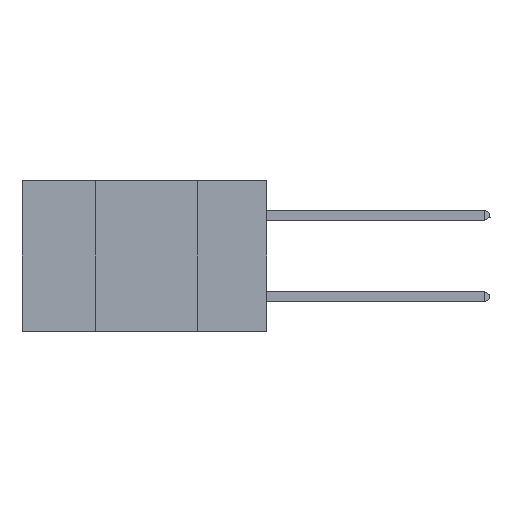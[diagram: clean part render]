
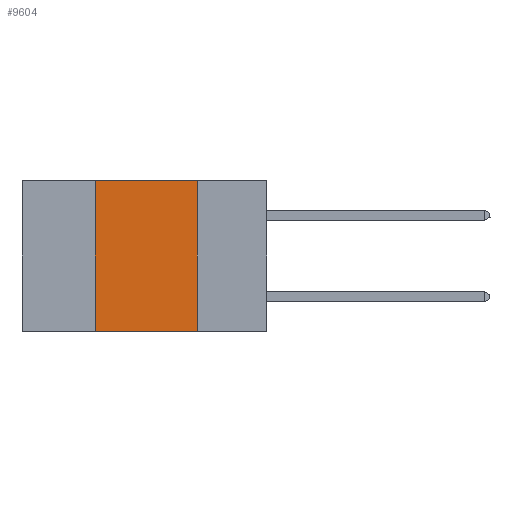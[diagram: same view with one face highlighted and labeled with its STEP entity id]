
A CAD part, left-side view. The second image highlights one B-rep face of the part: STEP entity #9604.
In plain terms, the highlighted planar face has unit normal (-1, 0, 0).
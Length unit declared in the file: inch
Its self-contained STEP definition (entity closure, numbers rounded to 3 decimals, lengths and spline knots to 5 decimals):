
#288 = CARTESIAN_POINT ( 'NONE',  ( 0., 0.6, -0.37 ) ) ;
#707 = VECTOR ( 'NONE', #19531, 39.37008 ) ;
#760 = CARTESIAN_POINT ( 'NONE',  ( 0., 0.17, -0.37 ) ) ;
#2148 = FACE_OUTER_BOUND ( 'NONE', #5654, .T. ) ;
#2434 = ORIENTED_EDGE ( 'NONE', *, *, #15368, .F. ) ;
#2664 = LINE ( 'NONE', #2764, #5301 ) ;
#2764 = CARTESIAN_POINT ( 'NONE',  ( 0., 0.42, 0. ) ) ;
#5301 = VECTOR ( 'NONE', #15510, 39.37008 ) ;
#5654 = EDGE_LOOP ( 'NONE', ( #12538, #9037, #2434, #13813 ) ) ;
#6790 = CARTESIAN_POINT ( 'NONE',  ( 0., 0.6, 0. ) ) ;
#7123 = LINE ( 'NONE', #288, #14876 ) ;
#8592 = CARTESIAN_POINT ( 'NONE',  ( 0., 0.17, 0. ) ) ;
#8779 = CARTESIAN_POINT ( 'NONE',  ( 0., 0.17, 0. ) ) ;
#9022 = LINE ( 'NONE', #8592, #707 ) ;
#9037 = ORIENTED_EDGE ( 'NONE', *, *, #16986, .F. ) ;
#9249 = AXIS2_PLACEMENT_3D ( 'NONE', #6790, #9571, #17397 ) ;
#9571 = DIRECTION ( 'NONE',  ( 1., 0., 0. ) ) ;
#9604 = ADVANCED_FACE ( 'NONE', ( #2148 ), #17537, .F. ) ;
#11187 = VERTEX_POINT ( 'NONE', #760 ) ;
#11320 = DIRECTION ( 'NONE',  ( 0., -1., 0. ) ) ;
#11720 = VERTEX_POINT ( 'NONE', #8779 ) ;
#12538 = ORIENTED_EDGE ( 'NONE', *, *, #17528, .F. ) ;
#13327 = VERTEX_POINT ( 'NONE', #15508 ) ;
#13466 = CARTESIAN_POINT ( 'NONE',  ( 0., 0.42, 0. ) ) ;
#13554 = VERTEX_POINT ( 'NONE', #13466 ) ;
#13813 = ORIENTED_EDGE ( 'NONE', *, *, #16169, .T. ) ;
#14082 = LINE ( 'NONE', #19841, #18985 ) ;
#14876 = VECTOR ( 'NONE', #11320, 39.37008 ) ;
#15368 = EDGE_CURVE ( 'NONE', #13327, #13554, #2664, .T. ) ;
#15508 = CARTESIAN_POINT ( 'NONE',  ( 0., 0.42, -0.37 ) ) ;
#15510 = DIRECTION ( 'NONE',  ( 0., 0., 1. ) ) ;
#16169 = EDGE_CURVE ( 'NONE', #13327, #11187, #7123, .T. ) ;
#16986 = EDGE_CURVE ( 'NONE', #13554, #11720, #14082, .T. ) ;
#17397 = DIRECTION ( 'NONE',  ( 0., 0., -1. ) ) ;
#17528 = EDGE_CURVE ( 'NONE', #11720, #11187, #9022, .T. ) ;
#17537 = PLANE ( 'NONE',  #9249 ) ;
#18985 = VECTOR ( 'NONE', #19903, 39.37008 ) ;
#19531 = DIRECTION ( 'NONE',  ( 0., 0., -1. ) ) ;
#19841 = CARTESIAN_POINT ( 'NONE',  ( 0., 0.6, 0. ) ) ;
#19903 = DIRECTION ( 'NONE',  ( 0., -1., 0. ) ) ;
